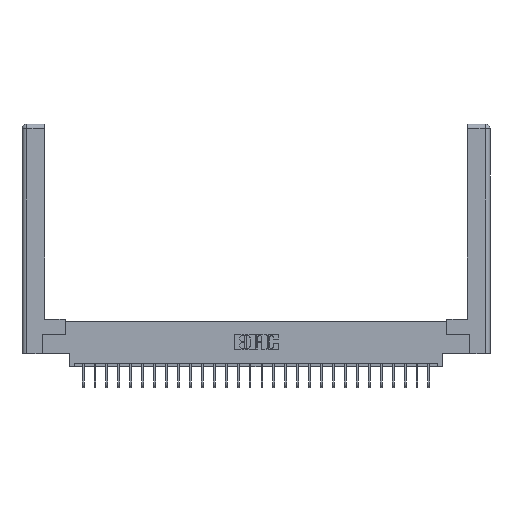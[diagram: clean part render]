
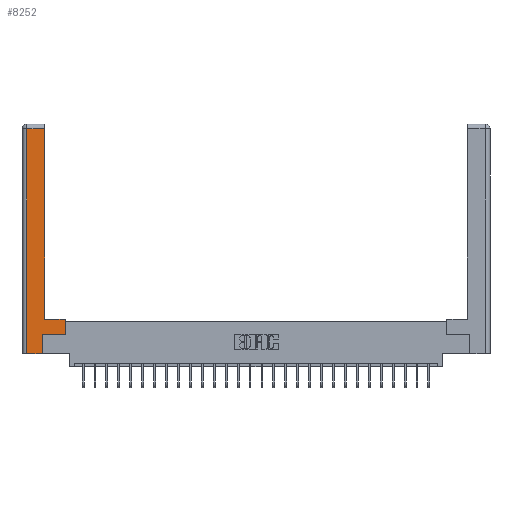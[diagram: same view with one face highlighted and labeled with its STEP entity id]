
A CAD part, top view. The second image highlights one B-rep face of the part: STEP entity #8252.
In plain terms, the highlighted planar face has unit normal (0, 0, 1).
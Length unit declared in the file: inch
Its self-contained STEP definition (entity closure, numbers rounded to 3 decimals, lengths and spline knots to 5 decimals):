
#154 = DIRECTION ( 'NONE',  ( -1., 0., 0. ) ) ;
#1333 = VECTOR ( 'NONE', #1722, 39.37008 ) ;
#1449 = ORIENTED_EDGE ( 'NONE', *, *, #24336, .T. ) ;
#1722 = DIRECTION ( 'NONE',  ( 0., 1., 0. ) ) ;
#2112 = AXIS2_PLACEMENT_3D ( 'NONE', #11131, #11030, #154 ) ;
#2276 = VERTEX_POINT ( 'NONE', #12931 ) ;
#3462 = CARTESIAN_POINT ( 'NONE',  ( 0.295, 3., 0. ) ) ;
#3470 = VECTOR ( 'NONE', #19964, 39.37008 ) ;
#3516 = LINE ( 'NONE', #29289, #12025 ) ;
#3802 = ORIENTED_EDGE ( 'NONE', *, *, #17985, .T. ) ;
#4531 = VECTOR ( 'NONE', #11798, 39.37008 ) ;
#4665 = EDGE_CURVE ( 'NONE', #4668, #27615, #29113, .T. ) ;
#4668 = VERTEX_POINT ( 'NONE', #19809 ) ;
#5738 = ORIENTED_EDGE ( 'NONE', *, *, #28713, .T. ) ;
#6752 = VERTEX_POINT ( 'NONE', #13695 ) ;
#8221 = CARTESIAN_POINT ( 'NONE',  ( 0.565, 0.45, 0. ) ) ;
#8249 = DIRECTION ( 'NONE',  ( 0., -1., 0. ) ) ;
#8252 = ADVANCED_FACE ( 'NONE', ( #10417 ), #22405, .F. ) ;
#9418 = CARTESIAN_POINT ( 'NONE',  ( 0.265, 0.245, 0. ) ) ;
#9457 = ORIENTED_EDGE ( 'NONE', *, *, #4665, .T. ) ;
#9623 = EDGE_CURVE ( 'NONE', #27615, #25285, #23731, .T. ) ;
#9850 = EDGE_CURVE ( 'NONE', #6752, #27957, #25478, .T. ) ;
#10417 = FACE_OUTER_BOUND ( 'NONE', #26096, .T. ) ;
#10561 = CARTESIAN_POINT ( 'NONE',  ( 0.0615, 0., 0. ) ) ;
#10625 = EDGE_CURVE ( 'NONE', #27957, #17496, #10817, .T. ) ;
#10817 = LINE ( 'NONE', #14300, #18651 ) ;
#11030 = DIRECTION ( 'NONE',  ( 0., 0., -1. ) ) ;
#11095 = DIRECTION ( 'NONE',  ( -1., 0., 0. ) ) ;
#11131 = CARTESIAN_POINT ( 'NONE',  ( 0., 0., 0. ) ) ;
#11326 = CARTESIAN_POINT ( 'NONE',  ( 0.265, 0.245, 0. ) ) ;
#11613 = LINE ( 'NONE', #12881, #3470 ) ;
#11798 = DIRECTION ( 'NONE',  ( 1., 0., 0. ) ) ;
#12025 = VECTOR ( 'NONE', #11095, 39.37008 ) ;
#12275 = ORIENTED_EDGE ( 'NONE', *, *, #10625, .T. ) ;
#12881 = CARTESIAN_POINT ( 'NONE',  ( 0.565, 0.245, 0. ) ) ;
#12931 = CARTESIAN_POINT ( 'NONE',  ( 0.295, 2.94, 0. ) ) ;
#13695 = CARTESIAN_POINT ( 'NONE',  ( 0.565, 0.245, 0. ) ) ;
#14087 = DIRECTION ( 'NONE',  ( 0., 1., 0. ) ) ;
#14300 = CARTESIAN_POINT ( 'NONE',  ( 0.295, 0.45, 0. ) ) ;
#14744 = ORIENTED_EDGE ( 'NONE', *, *, #9623, .T. ) ;
#15412 = LINE ( 'NONE', #9418, #21139 ) ;
#15670 = VERTEX_POINT ( 'NONE', #11326 ) ;
#16712 = DIRECTION ( 'NONE',  ( -1., 0., 0. ) ) ;
#17245 = DIRECTION ( 'NONE',  ( 0., 1., 0. ) ) ;
#17496 = VERTEX_POINT ( 'NONE', #25620 ) ;
#17714 = CARTESIAN_POINT ( 'NONE',  ( 0.0615, 0., 0. ) ) ;
#17985 = EDGE_CURVE ( 'NONE', #15670, #6752, #11613, .T. ) ;
#18574 = CARTESIAN_POINT ( 'NONE',  ( 0.265, 0., 0. ) ) ;
#18651 = VECTOR ( 'NONE', #16712, 39.37008 ) ;
#19809 = CARTESIAN_POINT ( 'NONE',  ( 0.0615, 2.94, 0. ) ) ;
#19964 = DIRECTION ( 'NONE',  ( 1., 0., 0. ) ) ;
#21139 = VECTOR ( 'NONE', #14087, 39.37008 ) ;
#22405 = PLANE ( 'NONE',  #2112 ) ;
#22805 = CARTESIAN_POINT ( 'NONE',  ( 0.565, 0.45, 0. ) ) ;
#22887 = LINE ( 'NONE', #3462, #23253 ) ;
#23253 = VECTOR ( 'NONE', #17245, 39.37008 ) ;
#23332 = CARTESIAN_POINT ( 'NONE',  ( 0.265, 0., 0. ) ) ;
#23452 = ORIENTED_EDGE ( 'NONE', *, *, #26812, .T. ) ;
#23731 = LINE ( 'NONE', #18574, #4531 ) ;
#24336 = EDGE_CURVE ( 'NONE', #2276, #4668, #3516, .T. ) ;
#24940 = ORIENTED_EDGE ( 'NONE', *, *, #9850, .T. ) ;
#25285 = VERTEX_POINT ( 'NONE', #23332 ) ;
#25478 = LINE ( 'NONE', #8221, #1333 ) ;
#25620 = CARTESIAN_POINT ( 'NONE',  ( 0.295, 0.45, 0. ) ) ;
#26096 = EDGE_LOOP ( 'NONE', ( #5738, #1449, #9457, #14744, #23452, #3802, #24940, #12275 ) ) ;
#26812 = EDGE_CURVE ( 'NONE', #25285, #15670, #15412, .T. ) ;
#26978 = VECTOR ( 'NONE', #8249, 39.37008 ) ;
#27615 = VERTEX_POINT ( 'NONE', #10561 ) ;
#27957 = VERTEX_POINT ( 'NONE', #22805 ) ;
#28713 = EDGE_CURVE ( 'NONE', #17496, #2276, #22887, .T. ) ;
#29113 = LINE ( 'NONE', #17714, #26978 ) ;
#29289 = CARTESIAN_POINT ( 'NONE',  ( 0.0615, 2.94, 0. ) ) ;
